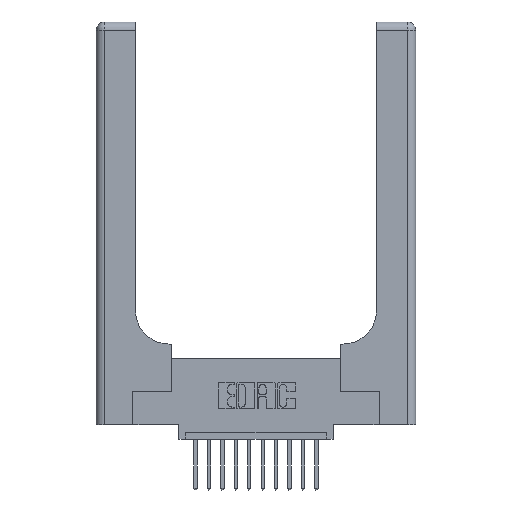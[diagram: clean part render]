
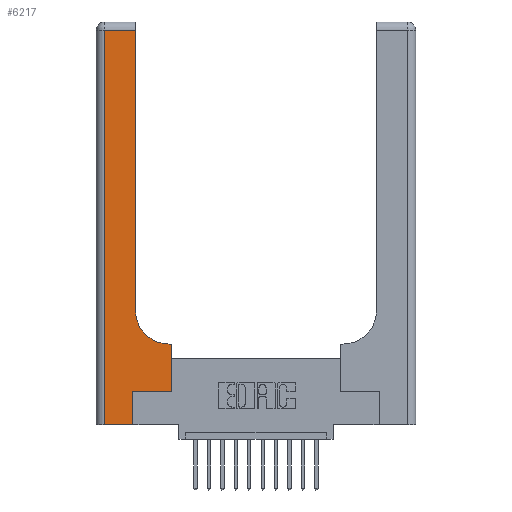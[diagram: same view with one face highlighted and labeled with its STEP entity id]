
A CAD part, top view. The second image highlights one B-rep face of the part: STEP entity #6217.
In plain terms, the highlighted planar face has unit normal (0, 0, 1).
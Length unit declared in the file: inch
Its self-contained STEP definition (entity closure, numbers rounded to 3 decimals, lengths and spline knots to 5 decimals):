
#8 = ORIENTED_EDGE ( 'NONE', *, *, #11506, .T. ) ;
#258 = PLANE ( 'NONE',  #2057 ) ;
#390 = CARTESIAN_POINT ( 'NONE',  ( 0.269, 0., 0.37 ) ) ;
#421 = EDGE_CURVE ( 'NONE', #7837, #14889, #9556, .T. ) ;
#423 = AXIS2_PLACEMENT_3D ( 'NONE', #9605, #544, #4521 ) ;
#544 = DIRECTION ( 'NONE',  ( 0., 0., -1. ) ) ;
#553 = VECTOR ( 'NONE', #15344, 39.37008 ) ;
#659 = CARTESIAN_POINT ( 'NONE',  ( 0.2915, 0.85, 0.37 ) ) ;
#797 = ORIENTED_EDGE ( 'NONE', *, *, #8925, .T. ) ;
#1063 = ORIENTED_EDGE ( 'NONE', *, *, #2394, .T. ) ;
#1650 = DIRECTION ( 'NONE',  ( -1., 0., 0. ) ) ;
#1760 = VERTEX_POINT ( 'NONE', #16164 ) ;
#1829 = DIRECTION ( 'NONE',  ( -1., 0., 0. ) ) ;
#2057 = AXIS2_PLACEMENT_3D ( 'NONE', #13686, #16342, #16226 ) ;
#2394 = EDGE_CURVE ( 'NONE', #4432, #7412, #4043, .T. ) ;
#2395 = VERTEX_POINT ( 'NONE', #390 ) ;
#2418 = VERTEX_POINT ( 'NONE', #15095 ) ;
#2911 = CARTESIAN_POINT ( 'NONE',  ( 0., 2.94, 0.37 ) ) ;
#3017 = CARTESIAN_POINT ( 'NONE',  ( 0.06, 0., 0.37 ) ) ;
#3623 = ORIENTED_EDGE ( 'NONE', *, *, #15887, .T. ) ;
#3742 = FACE_OUTER_BOUND ( 'NONE', #9370, .T. ) ;
#3991 = VECTOR ( 'NONE', #16223, 39.37008 ) ;
#4034 = LINE ( 'NONE', #2911, #11698 ) ;
#4043 = LINE ( 'NONE', #12605, #553 ) ;
#4210 = LINE ( 'NONE', #14728, #3991 ) ;
#4256 = VECTOR ( 'NONE', #9604, 39.37008 ) ;
#4432 = VERTEX_POINT ( 'NONE', #15271 ) ;
#4519 = ORIENTED_EDGE ( 'NONE', *, *, #14235, .T. ) ;
#4521 = DIRECTION ( 'NONE',  ( 1., 0., 0. ) ) ;
#4644 = CARTESIAN_POINT ( 'NONE',  ( 0.2915, 0.6, 0.37 ) ) ;
#4906 = ORIENTED_EDGE ( 'NONE', *, *, #16353, .T. ) ;
#5522 = ORIENTED_EDGE ( 'NONE', *, *, #13029, .T. ) ;
#5702 = VECTOR ( 'NONE', #14610, 39.37008 ) ;
#6217 = ADVANCED_FACE ( 'NONE', ( #3742 ), #258, .F. ) ;
#6999 = VECTOR ( 'NONE', #1829, 39.37008 ) ;
#7106 = CIRCLE ( 'NONE', #423, 0.25 ) ;
#7231 = VERTEX_POINT ( 'NONE', #15440 ) ;
#7412 = VERTEX_POINT ( 'NONE', #3017 ) ;
#7560 = LINE ( 'NONE', #7893, #5702 ) ;
#7837 = VERTEX_POINT ( 'NONE', #9149 ) ;
#7893 = CARTESIAN_POINT ( 'NONE',  ( 0.269, 0., 0.37 ) ) ;
#7979 = DIRECTION ( 'NONE',  ( 1., 0., 0. ) ) ;
#8234 = CARTESIAN_POINT ( 'NONE',  ( 0.2915, 3., 0.37 ) ) ;
#8809 = EDGE_CURVE ( 'NONE', #14889, #7231, #4210, .T. ) ;
#8925 = EDGE_CURVE ( 'NONE', #1760, #13035, #7106, .T. ) ;
#9109 = LINE ( 'NONE', #11168, #11177 ) ;
#9149 = CARTESIAN_POINT ( 'NONE',  ( 0.269, 0.25, 0.37 ) ) ;
#9370 = EDGE_LOOP ( 'NONE', ( #4906, #4519, #1063, #8, #3623, #17071, #9620, #5522, #797 ) ) ;
#9556 = LINE ( 'NONE', #17131, #17026 ) ;
#9604 = DIRECTION ( 'NONE',  ( 0., 1., 0. ) ) ;
#9605 = CARTESIAN_POINT ( 'NONE',  ( 0.5415, 0.85, 0.37 ) ) ;
#9620 = ORIENTED_EDGE ( 'NONE', *, *, #8809, .T. ) ;
#9939 = DIRECTION ( 'NONE',  ( 1., 0., 0. ) ) ;
#11168 = CARTESIAN_POINT ( 'NONE',  ( 0., 0., 0.37 ) ) ;
#11177 = VECTOR ( 'NONE', #9939, 39.37008 ) ;
#11506 = EDGE_CURVE ( 'NONE', #7412, #2395, #9109, .T. ) ;
#11698 = VECTOR ( 'NONE', #1650, 39.37008 ) ;
#12605 = CARTESIAN_POINT ( 'NONE',  ( 0.06, 3., 0.37 ) ) ;
#13029 = EDGE_CURVE ( 'NONE', #7231, #1760, #16725, .T. ) ;
#13035 = VERTEX_POINT ( 'NONE', #659 ) ;
#13686 = CARTESIAN_POINT ( 'NONE',  ( 0., 3., 0.37 ) ) ;
#14235 = EDGE_CURVE ( 'NONE', #2418, #4432, #4034, .T. ) ;
#14610 = DIRECTION ( 'NONE',  ( 0., 1., 0. ) ) ;
#14728 = CARTESIAN_POINT ( 'NONE',  ( 0.5585, 0.25, 0.37 ) ) ;
#14766 = CARTESIAN_POINT ( 'NONE',  ( 0.5585, 0.25, 0.37 ) ) ;
#14818 = LINE ( 'NONE', #8234, #4256 ) ;
#14889 = VERTEX_POINT ( 'NONE', #14766 ) ;
#15095 = CARTESIAN_POINT ( 'NONE',  ( 0.2915, 2.94, 0.37 ) ) ;
#15271 = CARTESIAN_POINT ( 'NONE',  ( 0.06, 2.94, 0.37 ) ) ;
#15344 = DIRECTION ( 'NONE',  ( 0., -1., 0. ) ) ;
#15440 = CARTESIAN_POINT ( 'NONE',  ( 0.5585, 0.6, 0.37 ) ) ;
#15887 = EDGE_CURVE ( 'NONE', #2395, #7837, #7560, .T. ) ;
#16164 = CARTESIAN_POINT ( 'NONE',  ( 0.5415, 0.6, 0.37 ) ) ;
#16223 = DIRECTION ( 'NONE',  ( 0., 1., 0. ) ) ;
#16226 = DIRECTION ( 'NONE',  ( -1., 0., 0. ) ) ;
#16342 = DIRECTION ( 'NONE',  ( 0., 0., -1. ) ) ;
#16353 = EDGE_CURVE ( 'NONE', #13035, #2418, #14818, .T. ) ;
#16725 = LINE ( 'NONE', #4644, #6999 ) ;
#17026 = VECTOR ( 'NONE', #7979, 39.37008 ) ;
#17071 = ORIENTED_EDGE ( 'NONE', *, *, #421, .T. ) ;
#17131 = CARTESIAN_POINT ( 'NONE',  ( 0.269, 0.25, 0.37 ) ) ;
